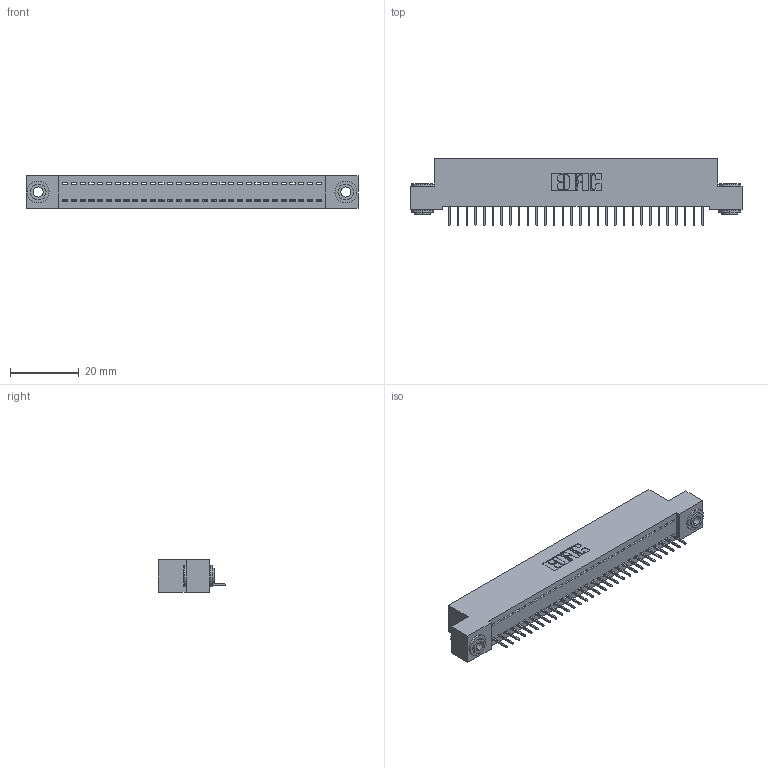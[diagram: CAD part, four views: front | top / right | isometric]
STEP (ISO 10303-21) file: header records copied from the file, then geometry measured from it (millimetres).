
FILE_DESCRIPTION (( 'STEP AP203' ), '1' );
FILE_NAME ('392-030-524-103.STEP', '2018-08-15T22:19:17', ( '' ), ( '' ), 'SwSTEP 2.0', 'SolidWorks 2016', '' );
FILE_SCHEMA (( 'CONFIG_CONTROL_DESIGN' ));
Length unit declared in the file: inch
Products named in the file (4): 345-292-001_345-293-124; 342-250-002_345-250-002-102; 392-030-524-103; 342 Part_.156 TH
Assembly tree (33 placements, depth 2):
  392-030-524-103
    342 Part_.156 TH
    345-292-001_345-293-124  x30
    342-250-002_345-250-002-102  x2
Bounding box: 96.52 x 19.69 x 9.4 mm (x, y, z)
Volume: 8323 mm3; surface area: 11855.9 mm2
Topology: 33 solids, 33 shells, 2008 faces, 5775 edges, 3726 vertices
Faces by surface type: plane 1516, cylinder 484, cone 8
Entity records: 20484 total; most frequent: CARTESIAN_POINT 3511, ORIENTED_EDGE 3470, DIRECTION 3021, EDGE_CURVE 1735, LINE 1587, VECTOR 1587, VERTEX_POINT 1150, AXIS2_PLACEMENT_3D 717
